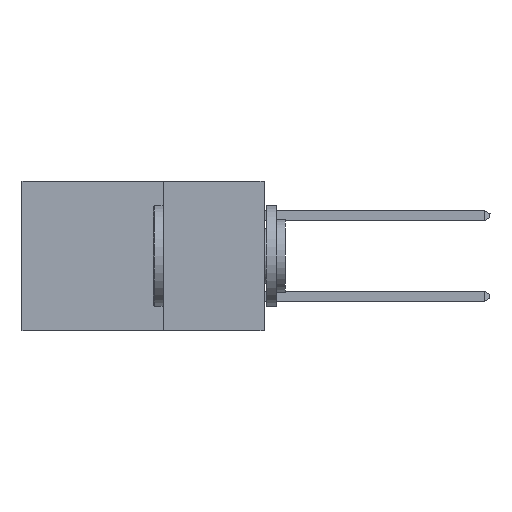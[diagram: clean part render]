
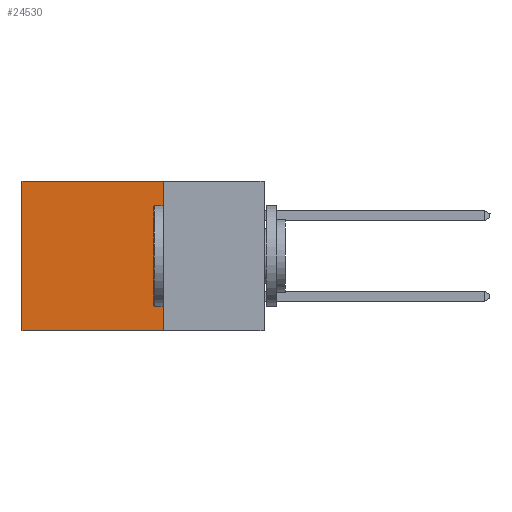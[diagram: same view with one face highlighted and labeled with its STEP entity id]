
A CAD part, left-side view. The second image highlights one B-rep face of the part: STEP entity #24530.
In plain terms, the highlighted planar face has unit normal (-1, 0, 0).
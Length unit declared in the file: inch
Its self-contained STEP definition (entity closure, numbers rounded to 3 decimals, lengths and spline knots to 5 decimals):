
#631 = LINE ( 'NONE', #13617, #23030 ) ;
#675 = CARTESIAN_POINT ( 'NONE',  ( 0.298, 0.6, -0.37 ) ) ;
#940 = DIRECTION ( 'NONE',  ( 0., 0., -1. ) ) ;
#2433 = EDGE_CURVE ( 'NONE', #12625, #14667, #3013, .T. ) ;
#3013 = LINE ( 'NONE', #11492, #14186 ) ;
#3176 = VECTOR ( 'NONE', #15961, 39.37008 ) ;
#5139 = CARTESIAN_POINT ( 'NONE',  ( 0.298, 0.6, 0. ) ) ;
#5781 = AXIS2_PLACEMENT_3D ( 'NONE', #26941, #12101, #940 ) ;
#5994 = VERTEX_POINT ( 'NONE', #13888 ) ;
#6855 = DIRECTION ( 'NONE',  ( 0., 1., 0. ) ) ;
#7237 = LINE ( 'NONE', #26204, #3176 ) ;
#7329 = ORIENTED_EDGE ( 'NONE', *, *, #7489, .F. ) ;
#7489 = EDGE_CURVE ( 'NONE', #5994, #20107, #12297, .T. ) ;
#8826 = CARTESIAN_POINT ( 'NONE',  ( 0.298, 0.25, -0.37 ) ) ;
#9340 = DIRECTION ( 'NONE',  ( 0., 0., -1. ) ) ;
#9420 = DIRECTION ( 'NONE',  ( 0., 1., 0. ) ) ;
#9749 = FACE_OUTER_BOUND ( 'NONE', #25459, .T. ) ;
#10247 = EDGE_CURVE ( 'NONE', #12625, #5994, #631, .T. ) ;
#11492 = CARTESIAN_POINT ( 'NONE',  ( 0.298, 0.25, 0. ) ) ;
#12101 = DIRECTION ( 'NONE',  ( 1., 0., 0. ) ) ;
#12297 = LINE ( 'NONE', #8826, #24587 ) ;
#12625 = VERTEX_POINT ( 'NONE', #26501 ) ;
#13617 = CARTESIAN_POINT ( 'NONE',  ( 0.298, 0.25, 0. ) ) ;
#13888 = CARTESIAN_POINT ( 'NONE',  ( 0.298, 0.25, -0.37 ) ) ;
#14186 = VECTOR ( 'NONE', #9420, 39.37008 ) ;
#14667 = VERTEX_POINT ( 'NONE', #5139 ) ;
#15961 = DIRECTION ( 'NONE',  ( 0., 0., -1. ) ) ;
#16339 = PLANE ( 'NONE',  #5781 ) ;
#16801 = ORIENTED_EDGE ( 'NONE', *, *, #25266, .T. ) ;
#20107 = VERTEX_POINT ( 'NONE', #675 ) ;
#22023 = ORIENTED_EDGE ( 'NONE', *, *, #2433, .T. ) ;
#23030 = VECTOR ( 'NONE', #9340, 39.37008 ) ;
#23059 = ORIENTED_EDGE ( 'NONE', *, *, #10247, .F. ) ;
#24530 = ADVANCED_FACE ( 'NONE', ( #9749 ), #16339, .F. ) ;
#24587 = VECTOR ( 'NONE', #6855, 39.37008 ) ;
#25266 = EDGE_CURVE ( 'NONE', #14667, #20107, #7237, .T. ) ;
#25459 = EDGE_LOOP ( 'NONE', ( #16801, #7329, #23059, #22023 ) ) ;
#26204 = CARTESIAN_POINT ( 'NONE',  ( 0.298, 0.6, 0. ) ) ;
#26501 = CARTESIAN_POINT ( 'NONE',  ( 0.298, 0.25, 0. ) ) ;
#26941 = CARTESIAN_POINT ( 'NONE',  ( 0.298, 0.25, 0. ) ) ;
